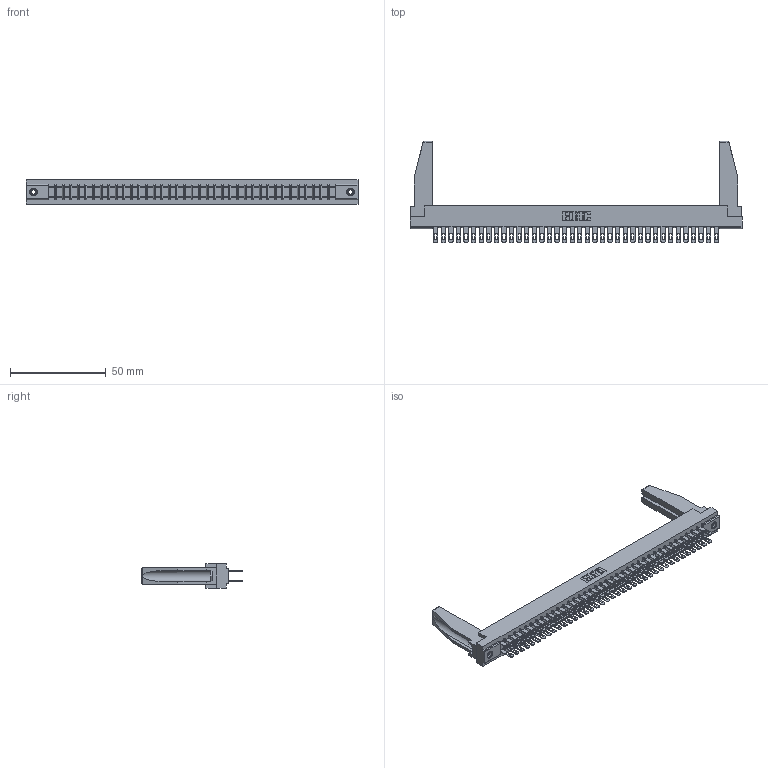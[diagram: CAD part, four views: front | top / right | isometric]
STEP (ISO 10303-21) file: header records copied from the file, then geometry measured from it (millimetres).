
FILE_DESCRIPTION (( 'STEP AP203' ), '1' );
FILE_NAME ('307-076-500-278.STEP', '2019-09-06T21:43:49', ( '' ), ( '' ), 'SwSTEP 2.0', 'SolidWorks 2016', '' );
FILE_SCHEMA (( 'CONFIG_CONTROL_DESIGN' ));
Length unit declared in the file: inch
Products named in the file (5): 307 Part_.156 Dia Mounting Holes; 307-220-078; 307-290-001_500; 307-076-500-278; 345-250-001_345-250-001-102
Assembly tree (81 placements, depth 2):
  307-076-500-278
    307 Part_.156 Dia Mounting Holes
    307-290-001_500  x76
    307-220-078  x2
    345-250-001_345-250-001-102  x2
Bounding box: 173.58 x 52.88 x 12.7 mm (x, y, z)
Volume: 22641.3 mm3; surface area: 27772.2 mm2
Topology: 81 solids, 81 shells, 3783 faces, 10533 edges, 6806 vertices
Faces by surface type: plane 2434, cylinder 1255, sphere 78, cone 12, torus 4
Entity records: 36699 total; most frequent: CARTESIAN_POINT 6012, ORIENTED_EDGE 5916, DIRECTION 5846, EDGE_CURVE 2958, LINE 2270, VECTOR 2270, VERTEX_POINT 1912, AXIS2_PLACEMENT_3D 1788
